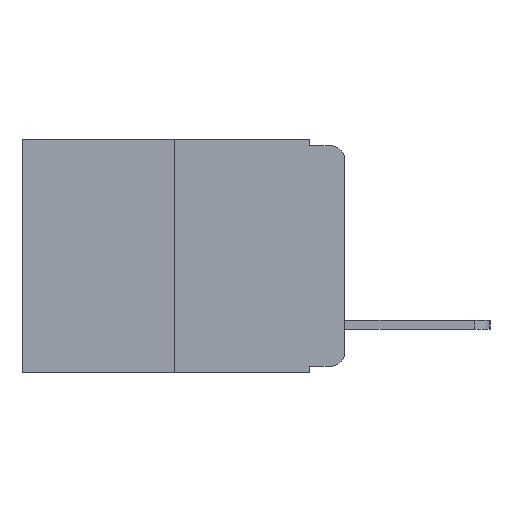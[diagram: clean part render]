
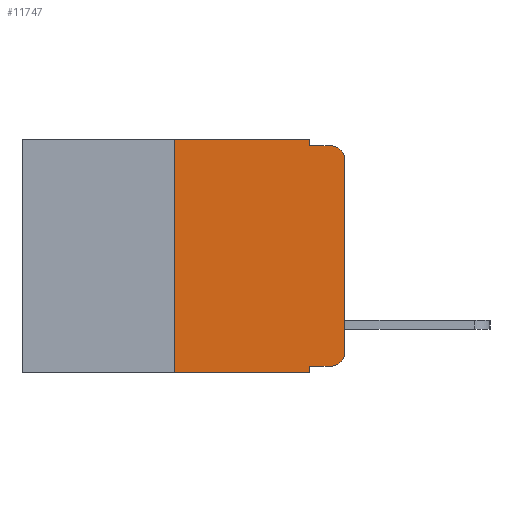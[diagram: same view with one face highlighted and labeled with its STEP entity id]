
A CAD part, left-side view. The second image highlights one B-rep face of the part: STEP entity #11747.
In plain terms, the highlighted planar face has unit normal (-1, 0, 0).
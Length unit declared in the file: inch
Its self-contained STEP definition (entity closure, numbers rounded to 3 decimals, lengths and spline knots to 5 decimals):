
#102 = VECTOR ( 'NONE', #5294, 39.37008 ) ;
#376 = EDGE_CURVE ( 'NONE', #2611, #1963, #11512, .T. ) ;
#456 = CARTESIAN_POINT ( 'NONE',  ( 0., 0.02, -0.333 ) ) ;
#505 = LINE ( 'NONE', #4093, #102 ) ;
#523 = AXIS2_PLACEMENT_3D ( 'NONE', #1019, #5995, #11713 ) ;
#664 = CARTESIAN_POINT ( 'NONE',  ( 0., 0.473, -0.343 ) ) ;
#1019 = CARTESIAN_POINT ( 'NONE',  ( 0., 0.473, 0. ) ) ;
#1090 = LINE ( 'NONE', #6367, #3526 ) ;
#1210 = DIRECTION ( 'NONE',  ( 0., 0., -1. ) ) ;
#1859 = DIRECTION ( 'NONE',  ( 0., 0., 1. ) ) ;
#1963 = VERTEX_POINT ( 'NONE', #9728 ) ;
#2064 = VECTOR ( 'NONE', #6954, 39.37008 ) ;
#2390 = CARTESIAN_POINT ( 'NONE',  ( 0., 0.02, -0.01 ) ) ;
#2608 = EDGE_CURVE ( 'NONE', #2611, #5616, #8990, .T. ) ;
#2611 = VERTEX_POINT ( 'NONE', #7016 ) ;
#2781 = CIRCLE ( 'NONE', #7090, 0.02 ) ;
#2880 = DIRECTION ( 'NONE',  ( 0., 0., -1. ) ) ;
#3090 = CARTESIAN_POINT ( 'NONE',  ( 0., 0.051, 0. ) ) ;
#3195 = CARTESIAN_POINT ( 'NONE',  ( 0., 0., 0. ) ) ;
#3421 = VERTEX_POINT ( 'NONE', #7891 ) ;
#3449 = DIRECTION ( 'NONE',  ( 0., 0., 1. ) ) ;
#3497 = DIRECTION ( 'NONE',  ( 0., -1., 0. ) ) ;
#3526 = VECTOR ( 'NONE', #1859, 39.37008 ) ;
#3585 = DIRECTION ( 'NONE',  ( 0., 0., -1. ) ) ;
#3704 = EDGE_LOOP ( 'NONE', ( #4914, #5052, #5327, #5257, #5468, #5518, #5788, #5720, #5796, #5954 ) ) ;
#3741 = CARTESIAN_POINT ( 'NONE',  ( 0., 0.25, 0. ) ) ;
#3753 = VECTOR ( 'NONE', #3585, 39.37008 ) ;
#3771 = CIRCLE ( 'NONE', #10424, 0.02 ) ;
#4010 = CARTESIAN_POINT ( 'NONE',  ( 0., 0.051, 0. ) ) ;
#4093 = CARTESIAN_POINT ( 'NONE',  ( 0., 0.051, -0.01 ) ) ;
#4408 = VERTEX_POINT ( 'NONE', #10374 ) ;
#4572 = LINE ( 'NONE', #664, #6713 ) ;
#4577 = VERTEX_POINT ( 'NONE', #10584 ) ;
#4873 = EDGE_CURVE ( 'NONE', #10696, #4408, #6948, .T. ) ;
#4914 = ORIENTED_EDGE ( 'NONE', *, *, #6326, .T. ) ;
#5052 = ORIENTED_EDGE ( 'NONE', *, *, #6901, .T. ) ;
#5072 = PLANE ( 'NONE',  #523 ) ;
#5074 = VERTEX_POINT ( 'NONE', #8052 ) ;
#5185 = VERTEX_POINT ( 'NONE', #2390 ) ;
#5257 = ORIENTED_EDGE ( 'NONE', *, *, #7320, .F. ) ;
#5294 = DIRECTION ( 'NONE',  ( 0., -1., 0. ) ) ;
#5305 = LINE ( 'NONE', #3195, #11642 ) ;
#5327 = ORIENTED_EDGE ( 'NONE', *, *, #7114, .F. ) ;
#5347 = CARTESIAN_POINT ( 'NONE',  ( 0., 0., -0.313 ) ) ;
#5468 = ORIENTED_EDGE ( 'NONE', *, *, #4873, .F. ) ;
#5518 = ORIENTED_EDGE ( 'NONE', *, *, #10060, .F. ) ;
#5616 = VERTEX_POINT ( 'NONE', #456 ) ;
#5720 = ORIENTED_EDGE ( 'NONE', *, *, #376, .F. ) ;
#5788 = ORIENTED_EDGE ( 'NONE', *, *, #9739, .T. ) ;
#5796 = ORIENTED_EDGE ( 'NONE', *, *, #2608, .T. ) ;
#5836 = CARTESIAN_POINT ( 'NONE',  ( 0., 0.02, -0.03 ) ) ;
#5954 = ORIENTED_EDGE ( 'NONE', *, *, #9970, .T. ) ;
#5957 = VERTEX_POINT ( 'NONE', #5347 ) ;
#5995 = DIRECTION ( 'NONE',  ( 1., 0., 0. ) ) ;
#6326 = EDGE_CURVE ( 'NONE', #5957, #4577, #5305, .T. ) ;
#6367 = CARTESIAN_POINT ( 'NONE',  ( 0., 0.25, 0. ) ) ;
#6436 = DIRECTION ( 'NONE',  ( -1., 0., 0. ) ) ;
#6713 = VECTOR ( 'NONE', #7571, 39.37008 ) ;
#6901 = EDGE_CURVE ( 'NONE', #4577, #5185, #3771, .T. ) ;
#6943 = CARTESIAN_POINT ( 'NONE',  ( 0., 0.051, -0.333 ) ) ;
#6948 = LINE ( 'NONE', #10214, #9162 ) ;
#6954 = DIRECTION ( 'NONE',  ( 0., -1., 0. ) ) ;
#7016 = CARTESIAN_POINT ( 'NONE',  ( 0., 0.051, -0.333 ) ) ;
#7090 = AXIS2_PLACEMENT_3D ( 'NONE', #11639, #11657, #1210 ) ;
#7114 = EDGE_CURVE ( 'NONE', #5074, #5185, #505, .T. ) ;
#7320 = EDGE_CURVE ( 'NONE', #4408, #5074, #10901, .T. ) ;
#7571 = DIRECTION ( 'NONE',  ( 0., -1., 0. ) ) ;
#7891 = CARTESIAN_POINT ( 'NONE',  ( 0., 0.25, -0.343 ) ) ;
#8052 = CARTESIAN_POINT ( 'NONE',  ( 0., 0.051, -0.01 ) ) ;
#8990 = LINE ( 'NONE', #6943, #2064 ) ;
#9162 = VECTOR ( 'NONE', #3497, 39.37008 ) ;
#9368 = DIRECTION ( 'NONE',  ( 0., 0., -1. ) ) ;
#9446 = VECTOR ( 'NONE', #9368, 39.37008 ) ;
#9728 = CARTESIAN_POINT ( 'NONE',  ( 0., 0.051, -0.343 ) ) ;
#9739 = EDGE_CURVE ( 'NONE', #3421, #1963, #4572, .T. ) ;
#9752 = FACE_OUTER_BOUND ( 'NONE', #3704, .T. ) ;
#9970 = EDGE_CURVE ( 'NONE', #5616, #5957, #2781, .T. ) ;
#10060 = EDGE_CURVE ( 'NONE', #3421, #10696, #1090, .T. ) ;
#10214 = CARTESIAN_POINT ( 'NONE',  ( 0., 0.473, 0. ) ) ;
#10374 = CARTESIAN_POINT ( 'NONE',  ( 0., 0.051, 0. ) ) ;
#10424 = AXIS2_PLACEMENT_3D ( 'NONE', #5836, #6436, #2880 ) ;
#10584 = CARTESIAN_POINT ( 'NONE',  ( 0., 0., -0.03 ) ) ;
#10696 = VERTEX_POINT ( 'NONE', #3741 ) ;
#10901 = LINE ( 'NONE', #3090, #3753 ) ;
#11512 = LINE ( 'NONE', #4010, #9446 ) ;
#11639 = CARTESIAN_POINT ( 'NONE',  ( 0., 0.02, -0.313 ) ) ;
#11642 = VECTOR ( 'NONE', #3449, 39.37008 ) ;
#11657 = DIRECTION ( 'NONE',  ( -1., 0., 0. ) ) ;
#11713 = DIRECTION ( 'NONE',  ( 0., 0., -1. ) ) ;
#11747 = ADVANCED_FACE ( 'NONE', ( #9752 ), #5072, .F. ) ;
